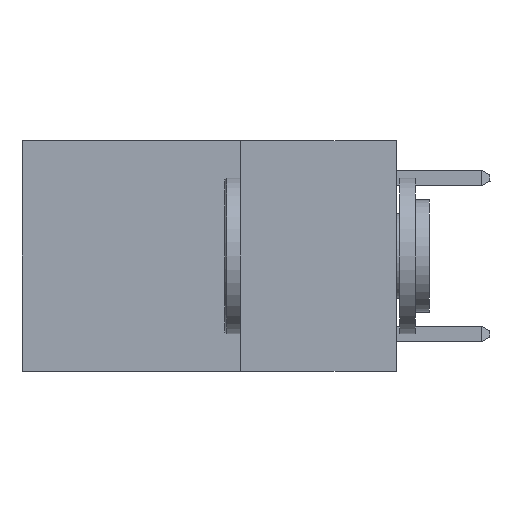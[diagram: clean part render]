
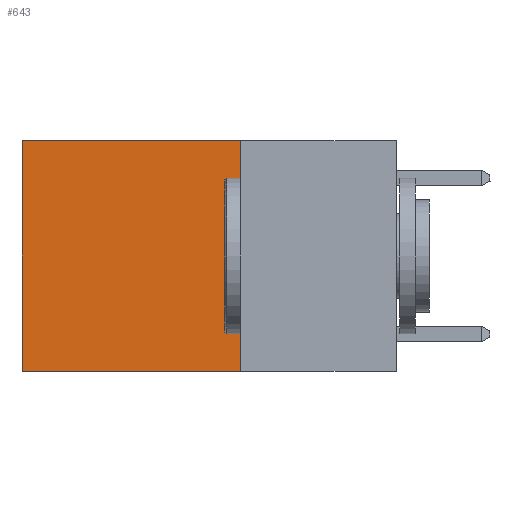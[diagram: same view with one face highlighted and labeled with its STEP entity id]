
A CAD part, left-side view. The second image highlights one B-rep face of the part: STEP entity #643.
In plain terms, the highlighted planar face has unit normal (-1, 0, 0).
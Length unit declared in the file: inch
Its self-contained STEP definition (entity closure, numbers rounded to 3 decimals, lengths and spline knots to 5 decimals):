
#155 = DIRECTION ( 'NONE',  ( 1., 0., 0. ) ) ;
#270 = CARTESIAN_POINT ( 'NONE',  ( 0.2625, 0.25, 0. ) ) ;
#416 = CARTESIAN_POINT ( 'NONE',  ( 0.2625, 0.25, 0. ) ) ;
#643 = ADVANCED_FACE ( 'NONE', ( #9255 ), #4508, .F. ) ;
#861 = CARTESIAN_POINT ( 'NONE',  ( 0.2625, 0.25, -0.37 ) ) ;
#1531 = DIRECTION ( 'NONE',  ( 0., 1., 0. ) ) ;
#1540 = CARTESIAN_POINT ( 'NONE',  ( 0.2625, 0.25, -0.37 ) ) ;
#1846 = ORIENTED_EDGE ( 'NONE', *, *, #4790, .T. ) ;
#1868 = EDGE_CURVE ( 'NONE', #6453, #2759, #8780, .T. ) ;
#1871 = ORIENTED_EDGE ( 'NONE', *, *, #1868, .T. ) ;
#2015 = EDGE_LOOP ( 'NONE', ( #1846, #7585, #4231, #1871 ) ) ;
#2759 = VERTEX_POINT ( 'NONE', #6251 ) ;
#3032 = LINE ( 'NONE', #861, #8832 ) ;
#3266 = CARTESIAN_POINT ( 'NONE',  ( 0.2625, 0.25, 0. ) ) ;
#3408 = VECTOR ( 'NONE', #6137, 39.37008 ) ;
#3439 = EDGE_CURVE ( 'NONE', #6453, #6182, #7648, .T. ) ;
#3719 = AXIS2_PLACEMENT_3D ( 'NONE', #8172, #155, #5244 ) ;
#4231 = ORIENTED_EDGE ( 'NONE', *, *, #3439, .F. ) ;
#4297 = LINE ( 'NONE', #7191, #8294 ) ;
#4508 = PLANE ( 'NONE',  #3719 ) ;
#4790 = EDGE_CURVE ( 'NONE', #2759, #5508, #4297, .T. ) ;
#4984 = DIRECTION ( 'NONE',  ( 0., 0., -1. ) ) ;
#5244 = DIRECTION ( 'NONE',  ( 0., 0., -1. ) ) ;
#5508 = VERTEX_POINT ( 'NONE', #6568 ) ;
#5810 = VECTOR ( 'NONE', #8539, 39.37008 ) ;
#6137 = DIRECTION ( 'NONE',  ( 0., 0., -1. ) ) ;
#6182 = VERTEX_POINT ( 'NONE', #1540 ) ;
#6251 = CARTESIAN_POINT ( 'NONE',  ( 0.2625, 0.6, 0. ) ) ;
#6453 = VERTEX_POINT ( 'NONE', #3266 ) ;
#6568 = CARTESIAN_POINT ( 'NONE',  ( 0.2625, 0.6, -0.37 ) ) ;
#7191 = CARTESIAN_POINT ( 'NONE',  ( 0.2625, 0.6, 0. ) ) ;
#7585 = ORIENTED_EDGE ( 'NONE', *, *, #7848, .F. ) ;
#7648 = LINE ( 'NONE', #270, #3408 ) ;
#7848 = EDGE_CURVE ( 'NONE', #6182, #5508, #3032, .T. ) ;
#8172 = CARTESIAN_POINT ( 'NONE',  ( 0.2625, 0.25, 0. ) ) ;
#8294 = VECTOR ( 'NONE', #4984, 39.37008 ) ;
#8539 = DIRECTION ( 'NONE',  ( 0., 1., 0. ) ) ;
#8780 = LINE ( 'NONE', #416, #5810 ) ;
#8832 = VECTOR ( 'NONE', #1531, 39.37008 ) ;
#9255 = FACE_OUTER_BOUND ( 'NONE', #2015, .T. ) ;
